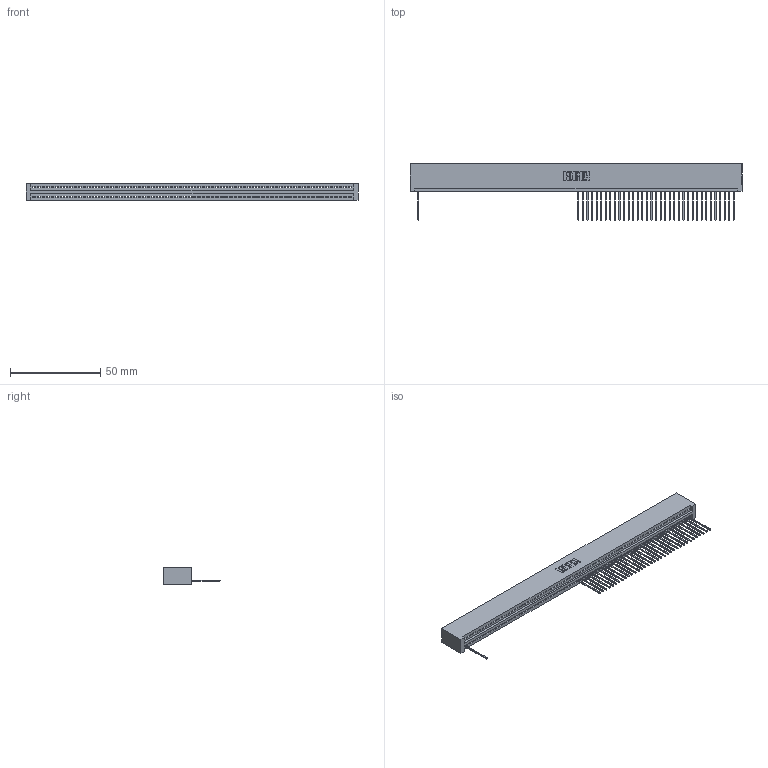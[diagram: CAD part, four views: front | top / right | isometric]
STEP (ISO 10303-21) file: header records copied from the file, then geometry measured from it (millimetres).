
FILE_DESCRIPTION (( 'STEP AP203' ), '1' );
FILE_NAME ('395-070-542-101.STEP', '2018-11-26T20:39:25', ( '' ), ( '' ), 'SwSTEP 2.0', 'SolidWorks 2016', '' );
FILE_SCHEMA (( 'CONFIG_CONTROL_DESIGN' ));
Length unit declared in the file: inch
Products named in the file (3): 345 Part_No Mounting Lugs; 395-070-542-101; 345-292-001_345-293-142
Assembly tree (37 placements, depth 2):
  395-070-542-101
    345 Part_No Mounting Lugs
    345-292-001_345-293-142  x36
Bounding box: 184.4 x 31.29 x 9.4 mm (x, y, z)
Volume: 18019.4 mm3; surface area: 22955.8 mm2
Topology: 37 solids, 37 shells, 2750 faces, 8489 edges, 5610 vertices
Faces by surface type: plane 1992, cylinder 758
Entity records: 47567 total; most frequent: ORIENTED_EDGE 8438, CARTESIAN_POINT 8400, DIRECTION 7251, EDGE_CURVE 4219, VECTOR 3815, LINE 3815, VERTEX_POINT 2810, AXIS2_PLACEMENT_3D 1718
